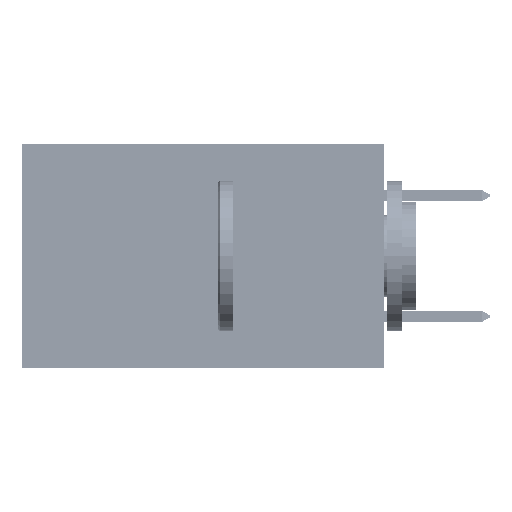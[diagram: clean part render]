
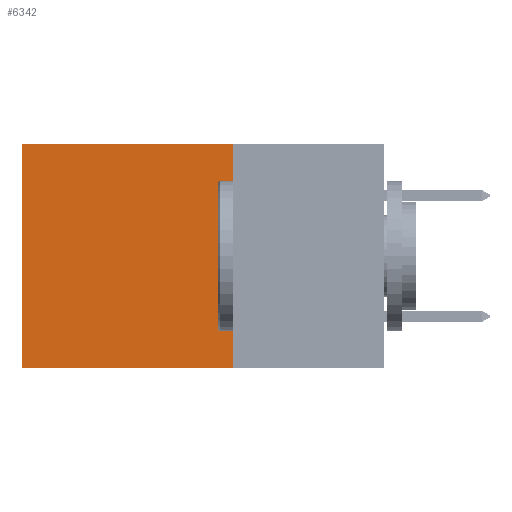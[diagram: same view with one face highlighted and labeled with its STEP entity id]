
A CAD part, left-side view. The second image highlights one B-rep face of the part: STEP entity #6342.
In plain terms, the highlighted planar face has unit normal (-1, 0, 0).
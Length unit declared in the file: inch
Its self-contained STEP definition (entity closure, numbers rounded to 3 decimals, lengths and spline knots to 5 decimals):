
#467 = EDGE_CURVE ( 'NONE', #23176, #38321, #3526, .T. ) ;
#2727 = CARTESIAN_POINT ( 'NONE',  ( 0.2875, 0.25, -0.37 ) ) ;
#3526 = LINE ( 'NONE', #17595, #39833 ) ;
#4353 = ORIENTED_EDGE ( 'NONE', *, *, #35168, .F. ) ;
#6342 = ADVANCED_FACE ( 'NONE', ( #40097 ), #39712, .F. ) ;
#6413 = VECTOR ( 'NONE', #32069, 39.37008 ) ;
#7142 = EDGE_LOOP ( 'NONE', ( #34124, #4353, #12949, #28794 ) ) ;
#7725 = LINE ( 'NONE', #2727, #17475 ) ;
#8708 = EDGE_CURVE ( 'NONE', #38321, #38757, #44754, .T. ) ;
#8991 = CARTESIAN_POINT ( 'NONE',  ( 0.2875, 0.25, 0. ) ) ;
#10994 = DIRECTION ( 'NONE',  ( 1., 0., 0. ) ) ;
#12949 = ORIENTED_EDGE ( 'NONE', *, *, #17711, .F. ) ;
#14313 = CARTESIAN_POINT ( 'NONE',  ( 0.2875, 0.6, 0. ) ) ;
#14600 = AXIS2_PLACEMENT_3D ( 'NONE', #25451, #10994, #36307 ) ;
#16578 = LINE ( 'NONE', #22539, #26232 ) ;
#17030 = DIRECTION ( 'NONE',  ( 0., 1., 0. ) ) ;
#17475 = VECTOR ( 'NONE', #28289, 39.37008 ) ;
#17595 = CARTESIAN_POINT ( 'NONE',  ( 0.2875, 0.25, 0. ) ) ;
#17711 = EDGE_CURVE ( 'NONE', #23176, #41942, #16578, .T. ) ;
#22539 = CARTESIAN_POINT ( 'NONE',  ( 0.2875, 0.25, 0. ) ) ;
#23176 = VERTEX_POINT ( 'NONE', #8991 ) ;
#24523 = CARTESIAN_POINT ( 'NONE',  ( 0.2875, 0.25, -0.37 ) ) ;
#25448 = CARTESIAN_POINT ( 'NONE',  ( 0.2875, 0.6, -0.37 ) ) ;
#25451 = CARTESIAN_POINT ( 'NONE',  ( 0.2875, 0.25, 0. ) ) ;
#26232 = VECTOR ( 'NONE', #36709, 39.37008 ) ;
#28289 = DIRECTION ( 'NONE',  ( 0., 1., 0. ) ) ;
#28794 = ORIENTED_EDGE ( 'NONE', *, *, #467, .T. ) ;
#32069 = DIRECTION ( 'NONE',  ( 0., 0., -1. ) ) ;
#34124 = ORIENTED_EDGE ( 'NONE', *, *, #8708, .T. ) ;
#35168 = EDGE_CURVE ( 'NONE', #41942, #38757, #7725, .T. ) ;
#35646 = CARTESIAN_POINT ( 'NONE',  ( 0.2875, 0.6, 0. ) ) ;
#36307 = DIRECTION ( 'NONE',  ( 0., 0., -1. ) ) ;
#36709 = DIRECTION ( 'NONE',  ( 0., 0., -1. ) ) ;
#38321 = VERTEX_POINT ( 'NONE', #14313 ) ;
#38757 = VERTEX_POINT ( 'NONE', #25448 ) ;
#39712 = PLANE ( 'NONE',  #14600 ) ;
#39833 = VECTOR ( 'NONE', #17030, 39.37008 ) ;
#40097 = FACE_OUTER_BOUND ( 'NONE', #7142, .T. ) ;
#41942 = VERTEX_POINT ( 'NONE', #24523 ) ;
#44754 = LINE ( 'NONE', #35646, #6413 ) ;
